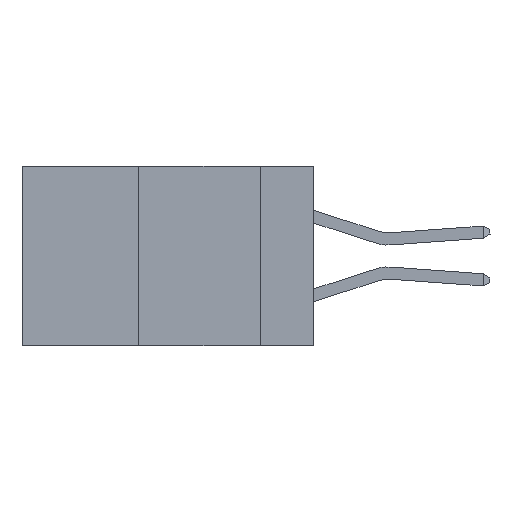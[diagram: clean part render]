
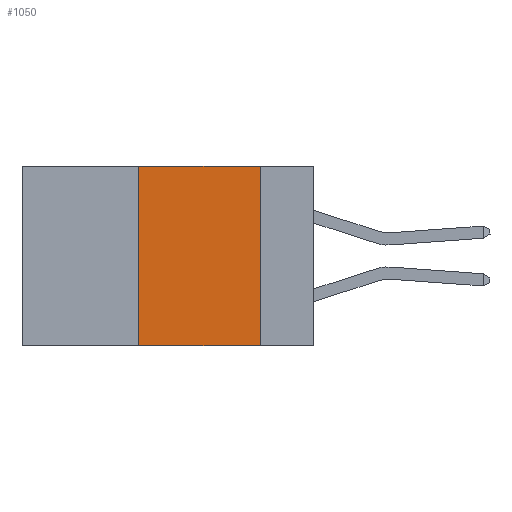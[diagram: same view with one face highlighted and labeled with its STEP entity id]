
A CAD part, left-side view. The second image highlights one B-rep face of the part: STEP entity #1050.
In plain terms, the highlighted planar face has unit normal (-1, 0, 0).
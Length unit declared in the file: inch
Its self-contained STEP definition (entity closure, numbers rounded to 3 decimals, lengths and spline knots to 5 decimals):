
#1050 = ADVANCED_FACE ( 'NONE', ( #9130 ), #37904, .F. ) ;
#1889 = CARTESIAN_POINT ( 'NONE',  ( 0., 0.11, 0. ) ) ;
#1943 = LINE ( 'NONE', #26132, #12684 ) ;
#2349 = LINE ( 'NONE', #14527, #34828 ) ;
#2479 = ORIENTED_EDGE ( 'NONE', *, *, #10482, .F. ) ;
#2601 = AXIS2_PLACEMENT_3D ( 'NONE', #31621, #9883, #22293 ) ;
#3739 = VECTOR ( 'NONE', #39049, 39.37008 ) ;
#4354 = ORIENTED_EDGE ( 'NONE', *, *, #27198, .F. ) ;
#6984 = CARTESIAN_POINT ( 'NONE',  ( 0., 0.11, -0.37 ) ) ;
#8421 = DIRECTION ( 'NONE',  ( 0., -1., 0. ) ) ;
#9130 = FACE_OUTER_BOUND ( 'NONE', #20716, .T. ) ;
#9883 = DIRECTION ( 'NONE',  ( 1., 0., 0. ) ) ;
#10029 = DIRECTION ( 'NONE',  ( 0., 0., 1. ) ) ;
#10482 = EDGE_CURVE ( 'NONE', #31406, #24124, #34812, .T. ) ;
#10610 = ORIENTED_EDGE ( 'NONE', *, *, #13522, .T. ) ;
#10885 = CARTESIAN_POINT ( 'NONE',  ( 0., 0.11, 0. ) ) ;
#12684 = VECTOR ( 'NONE', #8421, 39.37008 ) ;
#13098 = ORIENTED_EDGE ( 'NONE', *, *, #18672, .F. ) ;
#13522 = EDGE_CURVE ( 'NONE', #31406, #37316, #2349, .T. ) ;
#14527 = CARTESIAN_POINT ( 'NONE',  ( 0., 0.6, -0.37 ) ) ;
#16420 = CARTESIAN_POINT ( 'NONE',  ( 0., 0.36, -0.37 ) ) ;
#17131 = LINE ( 'NONE', #1889, #3739 ) ;
#18419 = VECTOR ( 'NONE', #10029, 39.37008 ) ;
#18672 = EDGE_CURVE ( 'NONE', #19458, #37316, #17131, .T. ) ;
#19458 = VERTEX_POINT ( 'NONE', #10885 ) ;
#20716 = EDGE_LOOP ( 'NONE', ( #13098, #4354, #2479, #10610 ) ) ;
#22293 = DIRECTION ( 'NONE',  ( 0., 0., -1. ) ) ;
#23508 = DIRECTION ( 'NONE',  ( 0., -1., 0. ) ) ;
#24124 = VERTEX_POINT ( 'NONE', #26739 ) ;
#26132 = CARTESIAN_POINT ( 'NONE',  ( 0., 0.6, 0. ) ) ;
#26739 = CARTESIAN_POINT ( 'NONE',  ( 0., 0.36, 0. ) ) ;
#27198 = EDGE_CURVE ( 'NONE', #24124, #19458, #1943, .T. ) ;
#28728 = CARTESIAN_POINT ( 'NONE',  ( 0., 0.36, 0. ) ) ;
#31406 = VERTEX_POINT ( 'NONE', #16420 ) ;
#31621 = CARTESIAN_POINT ( 'NONE',  ( 0., 0.6, 0. ) ) ;
#34812 = LINE ( 'NONE', #28728, #18419 ) ;
#34828 = VECTOR ( 'NONE', #23508, 39.37008 ) ;
#37316 = VERTEX_POINT ( 'NONE', #6984 ) ;
#37904 = PLANE ( 'NONE',  #2601 ) ;
#39049 = DIRECTION ( 'NONE',  ( 0., 0., -1. ) ) ;
